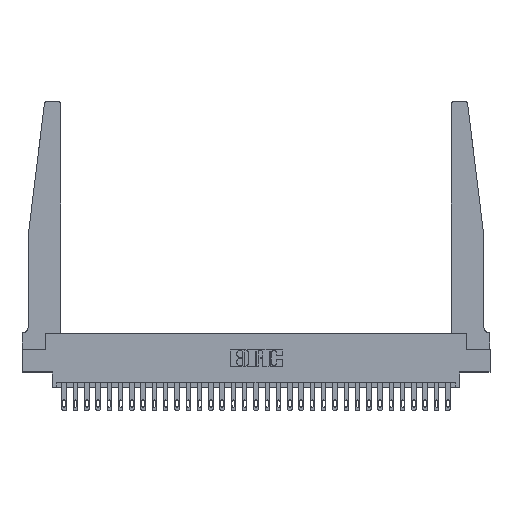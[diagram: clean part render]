
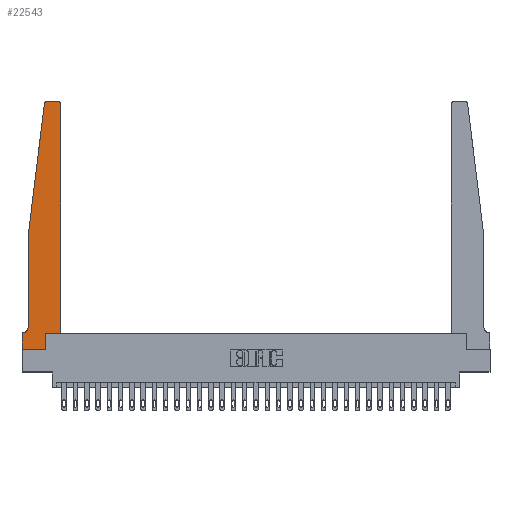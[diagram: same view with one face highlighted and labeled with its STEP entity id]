
A CAD part, top view. The second image highlights one B-rep face of the part: STEP entity #22543.
In plain terms, the highlighted planar face has unit normal (0, 0, 1).
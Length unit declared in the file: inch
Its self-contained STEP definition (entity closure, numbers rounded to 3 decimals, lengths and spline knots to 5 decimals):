
#130 = CARTESIAN_POINT ( 'NONE',  ( 0., 0., 0.37 ) ) ;
#188 = DIRECTION ( 'NONE',  ( -0.122, -0.992, 0. ) ) ;
#215 = VERTEX_POINT ( 'NONE', #11298 ) ;
#342 = ORIENTED_EDGE ( 'NONE', *, *, #11801, .T. ) ;
#460 = DIRECTION ( 'NONE',  ( 0., 0., 1. ) ) ;
#578 = LINE ( 'NONE', #9418, #11419 ) ;
#587 = CARTESIAN_POINT ( 'NONE',  ( 0., 0., 0.37 ) ) ;
#613 = ORIENTED_EDGE ( 'NONE', *, *, #24278, .T. ) ;
#672 = VECTOR ( 'NONE', #6571, 39.37008 ) ;
#895 = LINE ( 'NONE', #3102, #9886 ) ;
#1452 = CARTESIAN_POINT ( 'NONE',  ( 0., 0.1875, 0.37 ) ) ;
#1621 = ORIENTED_EDGE ( 'NONE', *, *, #26214, .T. ) ;
#2457 = EDGE_LOOP ( 'NONE', ( #342, #2941, #4101, #3263, #23387, #26550, #3666, #20257, #20768, #1621, #613, #19178 ) ) ;
#2941 = ORIENTED_EDGE ( 'NONE', *, *, #10453, .T. ) ;
#2974 = VERTEX_POINT ( 'NONE', #14541 ) ;
#3102 = CARTESIAN_POINT ( 'NONE',  ( 0.065, 1.25, 0.37 ) ) ;
#3113 = CARTESIAN_POINT ( 'NONE',  ( 0.25, 2.75, 0.37 ) ) ;
#3263 = ORIENTED_EDGE ( 'NONE', *, *, #4541, .T. ) ;
#3269 = CARTESIAN_POINT ( 'NONE',  ( 0.395, 2.72, 0.37 ) ) ;
#3666 = ORIENTED_EDGE ( 'NONE', *, *, #5912, .T. ) ;
#3886 = CIRCLE ( 'NONE', #12349, 0.03 ) ;
#4089 = EDGE_CURVE ( 'NONE', #2974, #22504, #11390, .T. ) ;
#4101 = ORIENTED_EDGE ( 'NONE', *, *, #4089, .T. ) ;
#4430 = DIRECTION ( 'NONE',  ( 0., 0., 1. ) ) ;
#4541 = EDGE_CURVE ( 'NONE', #22504, #4600, #895, .T. ) ;
#4600 = VERTEX_POINT ( 'NONE', #14137 ) ;
#5912 = EDGE_CURVE ( 'NONE', #26041, #22199, #7210, .T. ) ;
#6420 = DIRECTION ( 'NONE',  ( 0., 0., -1. ) ) ;
#6571 = DIRECTION ( 'NONE',  ( -1., 0., 0. ) ) ;
#6954 = DIRECTION ( 'NONE',  ( 1., 0., 0. ) ) ;
#7210 = LINE ( 'NONE', #587, #28687 ) ;
#9010 = VERTEX_POINT ( 'NONE', #13136 ) ;
#9270 = DIRECTION ( 'NONE',  ( 1., 0., 0. ) ) ;
#9418 = CARTESIAN_POINT ( 'NONE',  ( 0.425, 0.18, 0.37 ) ) ;
#9432 = DIRECTION ( 'NONE',  ( 1., 0., 0. ) ) ;
#9549 = VERTEX_POINT ( 'NONE', #13637 ) ;
#9765 = LINE ( 'NONE', #18761, #22017 ) ;
#9886 = VECTOR ( 'NONE', #25341, 39.37008 ) ;
#10015 = DIRECTION ( 'NONE',  ( -1., 0., 0. ) ) ;
#10139 = CARTESIAN_POINT ( 'NONE',  ( 0.065, 1.25, 0.37 ) ) ;
#10434 = DIRECTION ( 'NONE',  ( 0., 0., 1. ) ) ;
#10453 = EDGE_CURVE ( 'NONE', #9010, #2974, #25122, .T. ) ;
#10601 = LINE ( 'NONE', #28676, #17082 ) ;
#10727 = EDGE_CURVE ( 'NONE', #17822, #215, #10601, .T. ) ;
#11034 = VECTOR ( 'NONE', #10015, 39.37008 ) ;
#11298 = CARTESIAN_POINT ( 'NONE',  ( 0.2605, 0.18, 0.37 ) ) ;
#11390 = LINE ( 'NONE', #13456, #28656 ) ;
#11419 = VECTOR ( 'NONE', #9270, 39.37008 ) ;
#11801 = EDGE_CURVE ( 'NONE', #24333, #9010, #22855, .T. ) ;
#12007 = CARTESIAN_POINT ( 'NONE',  ( 0.395, 2.75, 0.37 ) ) ;
#12347 = CARTESIAN_POINT ( 'NONE',  ( 0.2605, 0., 0.37 ) ) ;
#12349 = AXIS2_PLACEMENT_3D ( 'NONE', #3269, #460, #9432 ) ;
#12657 = FACE_OUTER_BOUND ( 'NONE', #2457, .T. ) ;
#13136 = CARTESIAN_POINT ( 'NONE',  ( 0.27653, 2.75, 0.37 ) ) ;
#13456 = CARTESIAN_POINT ( 'NONE',  ( 0.065, 1.25, 0.37 ) ) ;
#13637 = CARTESIAN_POINT ( 'NONE',  ( 0.425, 0.18, 0.37 ) ) ;
#13846 = CARTESIAN_POINT ( 'NONE',  ( 0.27653, 2.72, 0.37 ) ) ;
#13897 = LINE ( 'NONE', #24543, #672 ) ;
#14137 = CARTESIAN_POINT ( 'NONE',  ( 0.065, 0.2375, 0.37 ) ) ;
#14424 = EDGE_CURVE ( 'NONE', #19716, #24333, #3886, .T. ) ;
#14541 = CARTESIAN_POINT ( 'NONE',  ( 0.24675, 2.72367, 0.37 ) ) ;
#15053 = EDGE_CURVE ( 'NONE', #16895, #26041, #13897, .T. ) ;
#15207 = EDGE_CURVE ( 'NONE', #4600, #16895, #17619, .T. ) ;
#15948 = CARTESIAN_POINT ( 'NONE',  ( 0., 0., 0.37 ) ) ;
#16895 = VERTEX_POINT ( 'NONE', #23782 ) ;
#17082 = VECTOR ( 'NONE', #28244, 39.37008 ) ;
#17619 = CIRCLE ( 'NONE', #18570, 0.05 ) ;
#17822 = VERTEX_POINT ( 'NONE', #12347 ) ;
#17920 = DIRECTION ( 'NONE',  ( -1., 0., 0. ) ) ;
#18153 = LINE ( 'NONE', #15948, #21577 ) ;
#18570 = AXIS2_PLACEMENT_3D ( 'NONE', #26608, #6420, #17920 ) ;
#18761 = CARTESIAN_POINT ( 'NONE',  ( 0.425, 0.18, 0.37 ) ) ;
#19178 = ORIENTED_EDGE ( 'NONE', *, *, #14424, .T. ) ;
#19413 = DIRECTION ( 'NONE',  ( 1., 0., 0. ) ) ;
#19716 = VERTEX_POINT ( 'NONE', #24803 ) ;
#20257 = ORIENTED_EDGE ( 'NONE', *, *, #24741, .T. ) ;
#20768 = ORIENTED_EDGE ( 'NONE', *, *, #10727, .T. ) ;
#21577 = VECTOR ( 'NONE', #6954, 39.37008 ) ;
#21634 = PLANE ( 'NONE',  #26640 ) ;
#22017 = VECTOR ( 'NONE', #27726, 39.37008 ) ;
#22199 = VERTEX_POINT ( 'NONE', #130 ) ;
#22264 = DIRECTION ( 'NONE',  ( 1., 0., 0. ) ) ;
#22288 = AXIS2_PLACEMENT_3D ( 'NONE', #13846, #4430, #22264 ) ;
#22504 = VERTEX_POINT ( 'NONE', #10139 ) ;
#22543 = ADVANCED_FACE ( 'NONE', ( #12657 ), #21634, .T. ) ;
#22855 = LINE ( 'NONE', #3113, #11034 ) ;
#23387 = ORIENTED_EDGE ( 'NONE', *, *, #15207, .T. ) ;
#23782 = CARTESIAN_POINT ( 'NONE',  ( 0.015, 0.1875, 0.37 ) ) ;
#24278 = EDGE_CURVE ( 'NONE', #9549, #19716, #9765, .T. ) ;
#24333 = VERTEX_POINT ( 'NONE', #12007 ) ;
#24543 = CARTESIAN_POINT ( 'NONE',  ( 0.065, 0.1875, 0.37 ) ) ;
#24741 = EDGE_CURVE ( 'NONE', #22199, #17822, #18153, .T. ) ;
#24803 = CARTESIAN_POINT ( 'NONE',  ( 0.425, 2.72, 0.37 ) ) ;
#25122 = CIRCLE ( 'NONE', #22288, 0.03 ) ;
#25341 = DIRECTION ( 'NONE',  ( 0., -1., 0. ) ) ;
#25484 = DIRECTION ( 'NONE',  ( 0., -1., 0. ) ) ;
#26041 = VERTEX_POINT ( 'NONE', #26797 ) ;
#26214 = EDGE_CURVE ( 'NONE', #215, #9549, #578, .T. ) ;
#26550 = ORIENTED_EDGE ( 'NONE', *, *, #15053, .T. ) ;
#26608 = CARTESIAN_POINT ( 'NONE',  ( 0.015, 0.2375, 0.37 ) ) ;
#26640 = AXIS2_PLACEMENT_3D ( 'NONE', #1452, #10434, #19413 ) ;
#26797 = CARTESIAN_POINT ( 'NONE',  ( 0., 0.1875, 0.37 ) ) ;
#27726 = DIRECTION ( 'NONE',  ( 0., 1., 0. ) ) ;
#28244 = DIRECTION ( 'NONE',  ( 0., 1., 0. ) ) ;
#28656 = VECTOR ( 'NONE', #188, 39.37008 ) ;
#28676 = CARTESIAN_POINT ( 'NONE',  ( 0.2605, 0.18, 0.37 ) ) ;
#28687 = VECTOR ( 'NONE', #25484, 39.37008 ) ;
